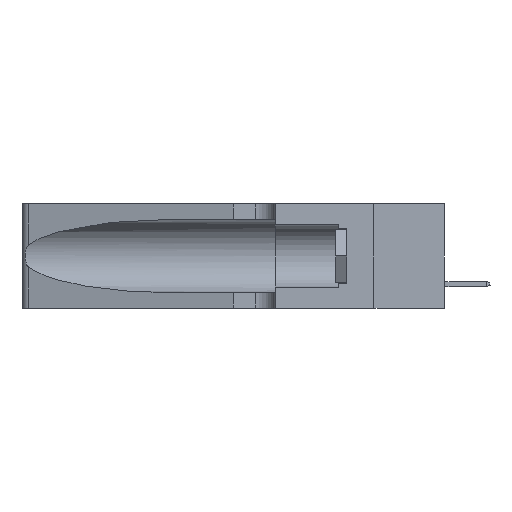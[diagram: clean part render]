
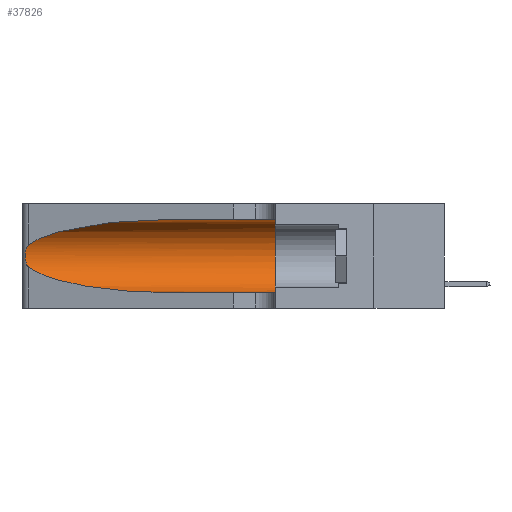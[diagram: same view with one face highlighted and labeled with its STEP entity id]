
A CAD part, left-side view. The second image highlights one B-rep face of the part: STEP entity #37826.
In plain terms, the highlighted cylindrical face has radius 3.308 mm (diameter 6.617 mm), a partial arc.
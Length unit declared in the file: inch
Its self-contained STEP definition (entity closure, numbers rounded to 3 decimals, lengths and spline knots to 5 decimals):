
#183 = CARTESIAN_POINT ( 'NONE',  ( 0.25487, 1.22718, 0.14631 ) ) ;
#778 = CARTESIAN_POINT ( 'NONE',  ( 0.25487, 1.22718, 0.22369 ) ) ;
#956 = VERTEX_POINT ( 'NONE', #38051 ) ;
#1825 = CARTESIAN_POINT ( 'NONE',  ( 0.2373, 1.15595, 0.28018 ) ) ;
#6131 = ORIENTED_EDGE ( 'NONE', *, *, #39028, .T. ) ;
#6674 = DIRECTION ( 'NONE',  ( 0., 1., 0. ) ) ;
#8911 = CARTESIAN_POINT ( 'NONE',  ( 0.25854, 1.2359, 0.20912 ) ) ;
#9204 = CARTESIAN_POINT ( 'NONE',  ( 0.1305, 1.61858, 0.31525 ) ) ;
#9556 = CARTESIAN_POINT ( 'NONE',  ( 0.18966, 0.96281, 0.05475 ) ) ;
#9675 = CARTESIAN_POINT ( 'NONE',  ( 0.2373, 1.15595, 0.08982 ) ) ;
#9728 = EDGE_CURVE ( 'NONE', #29826, #35203, #28050, .T. ) ;
#10275 = CARTESIAN_POINT ( 'NONE',  ( 0.25555, 1.22994, 0.2215 ) ) ;
#11262 = CARTESIAN_POINT ( 'NONE',  ( 0.25487, 1.22718, 0.22369 ) ) ;
#11684 = VERTEX_POINT ( 'NONE', #33478 ) ;
#12419 = CARTESIAN_POINT ( 'NONE',  ( 0.1305, 1.61858, 0.05475 ) ) ;
#12539 = DIRECTION ( 'NONE',  ( 0., -1., 0. ) ) ;
#13132 = ORIENTED_EDGE ( 'NONE', *, *, #33343, .F. ) ;
#13261 = CARTESIAN_POINT ( 'NONE',  ( 0.1305, 0.35, 0.185 ) ) ;
#13329 = VECTOR ( 'NONE', #28758, 39.37008 ) ;
#14852 = CARTESIAN_POINT ( 'NONE',  ( 0.1305, 0.72297, 0.31525 ) ) ;
#15055 = CARTESIAN_POINT ( 'NONE',  ( 0.25787, 1.23484, 0.2124 ) ) ;
#15070 = DIRECTION ( 'NONE',  ( 0., -1., 0. ) ) ;
#15183 = B_SPLINE_CURVE_WITH_KNOTS ( 'NONE', 3,
 ( #778, #10275, #36948, #15055, #8911, #34581, #15468, #37378, #21554, #34852, #22234, #25582, #34718, #18868 ),
 .UNSPECIFIED., .F., .F.,
 ( 4, 2, 2, 2, 2, 2, 4 ),
 ( 0., 0.00027, 0.00053, 0.00107, 0.0016, 0.00187, 0.00214 ),
 .UNSPECIFIED. ) ;
#15456 = CARTESIAN_POINT ( 'NONE',  ( 0.1305, 0.35, 0.31525 ) ) ;
#15468 = CARTESIAN_POINT ( 'NONE',  ( 0.26075, 1.23896, 0.19203 ) ) ;
#15695 = AXIS2_PLACEMENT_3D ( 'NONE', #13261, #6674, #19736 ) ;
#15803 = AXIS2_PLACEMENT_3D ( 'NONE', #28610, #12539, #18987 ) ;
#15805 = CYLINDRICAL_SURFACE ( 'NONE', #15803, 0.13025 ) ;
#16180 = LINE ( 'NONE', #12419, #39140 ) ;
#18868 = CARTESIAN_POINT ( 'NONE',  ( 0.25487, 1.22718, 0.14631 ) ) ;
#18987 = DIRECTION ( 'NONE',  ( 0., 0., -1. ) ) ;
#19037 = EDGE_LOOP ( 'NONE', ( #25244, #32732, #6131, #21413, #21095, #13132 ) ) ;
#19736 = DIRECTION ( 'NONE',  ( 0., 0., 1. ) ) ;
#21017 = CARTESIAN_POINT ( 'NONE',  ( 0.18966, 0.96281, 0.31525 ) ) ;
#21095 = ORIENTED_EDGE ( 'NONE', *, *, #33069, .F. ) ;
#21413 = ORIENTED_EDGE ( 'NONE', *, *, #26494, .T. ) ;
#21554 = CARTESIAN_POINT ( 'NONE',  ( 0.26017, 1.23833, 0.17102 ) ) ;
#21998 = CIRCLE ( 'NONE', #15695, 0.13025 ) ;
#22234 = CARTESIAN_POINT ( 'NONE',  ( 0.25789, 1.23486, 0.15765 ) ) ;
#22630 =( BOUNDED_CURVE ( )  B_SPLINE_CURVE ( 3, ( #183, #9675, #9556, #32024 ),
 .UNSPECIFIED., .F., .F. ) 
 B_SPLINE_CURVE_WITH_KNOTS ( ( 4, 4 ),
 ( 3.44316, 4.71239 ),
 .UNSPECIFIED. ) 
 CURVE ( )  GEOMETRIC_REPRESENTATION_ITEM ( )  RATIONAL_B_SPLINE_CURVE ( ( 1., 0.87, 0.87, 1. ) ) 
 REPRESENTATION_ITEM ( '' )  );
#25244 = ORIENTED_EDGE ( 'NONE', *, *, #9728, .T. ) ;
#25582 = CARTESIAN_POINT ( 'NONE',  ( 0.25639, 1.23186, 0.15144 ) ) ;
#26494 = EDGE_CURVE ( 'NONE', #956, #11684, #16180, .T. ) ;
#27570 = CARTESIAN_POINT ( 'NONE',  ( 0.1305, 0.72297, 0.31525 ) ) ;
#27774 = CARTESIAN_POINT ( 'NONE',  ( 0.25487, 1.22718, 0.14631 ) ) ;
#28050 =( BOUNDED_CURVE ( )  B_SPLINE_CURVE ( 3, ( #27570, #21017, #1825, #36977 ),
 .UNSPECIFIED., .F., .T. ) 
 B_SPLINE_CURVE_WITH_KNOTS ( ( 4, 4 ),
 ( 1.5708, 2.84003 ),
 .UNSPECIFIED. ) 
 CURVE ( )  GEOMETRIC_REPRESENTATION_ITEM ( )  RATIONAL_B_SPLINE_CURVE ( ( 1., 0.87, 0.87, 1. ) ) 
 REPRESENTATION_ITEM ( '' )  );
#28610 = CARTESIAN_POINT ( 'NONE',  ( 0.1305, 1.61858, 0.185 ) ) ;
#28758 = DIRECTION ( 'NONE',  ( 0., -1., 0. ) ) ;
#29826 = VERTEX_POINT ( 'NONE', #14852 ) ;
#30973 = EDGE_CURVE ( 'NONE', #35203, #38813, #15183, .T. ) ;
#32024 = CARTESIAN_POINT ( 'NONE',  ( 0.1305, 0.72297, 0.05475 ) ) ;
#32732 = ORIENTED_EDGE ( 'NONE', *, *, #30973, .T. ) ;
#33069 = EDGE_CURVE ( 'NONE', #34885, #11684, #21998, .T. ) ;
#33343 = EDGE_CURVE ( 'NONE', #29826, #34885, #39842, .T. ) ;
#33478 = CARTESIAN_POINT ( 'NONE',  ( 0.1305, 0.35, 0.05475 ) ) ;
#34581 = CARTESIAN_POINT ( 'NONE',  ( 0.26018, 1.23835, 0.19895 ) ) ;
#34718 = CARTESIAN_POINT ( 'NONE',  ( 0.25555, 1.22993, 0.14849 ) ) ;
#34852 = CARTESIAN_POINT ( 'NONE',  ( 0.25856, 1.23593, 0.16098 ) ) ;
#34885 = VERTEX_POINT ( 'NONE', #15456 ) ;
#35203 = VERTEX_POINT ( 'NONE', #11262 ) ;
#36948 = CARTESIAN_POINT ( 'NONE',  ( 0.25639, 1.23184, 0.21858 ) ) ;
#36977 = CARTESIAN_POINT ( 'NONE',  ( 0.25487, 1.22718, 0.22369 ) ) ;
#37378 = CARTESIAN_POINT ( 'NONE',  ( 0.26075, 1.23896, 0.178 ) ) ;
#37826 = ADVANCED_FACE ( 'NONE', ( #39204 ), #15805, .F. ) ;
#38051 = CARTESIAN_POINT ( 'NONE',  ( 0.1305, 0.72297, 0.05475 ) ) ;
#38813 = VERTEX_POINT ( 'NONE', #27774 ) ;
#39028 = EDGE_CURVE ( 'NONE', #38813, #956, #22630, .T. ) ;
#39140 = VECTOR ( 'NONE', #15070, 39.37008 ) ;
#39204 = FACE_OUTER_BOUND ( 'NONE', #19037, .T. ) ;
#39842 = LINE ( 'NONE', #9204, #13329 ) ;
